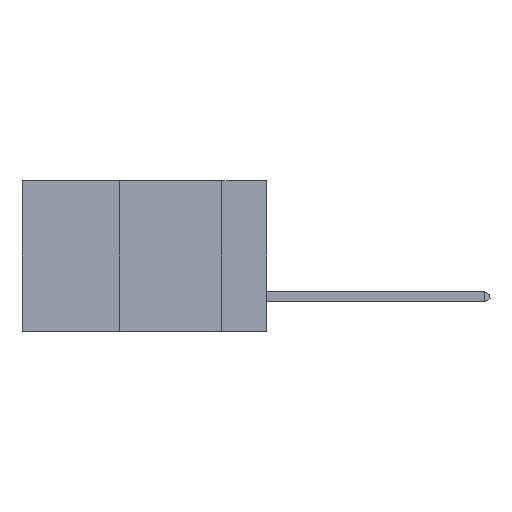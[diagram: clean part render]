
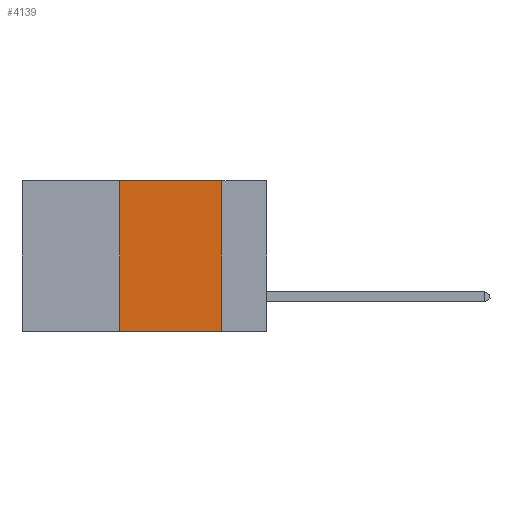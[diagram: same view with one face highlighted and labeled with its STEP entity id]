
A CAD part, left-side view. The second image highlights one B-rep face of the part: STEP entity #4139.
In plain terms, the highlighted planar face has unit normal (-1, 0, 0).
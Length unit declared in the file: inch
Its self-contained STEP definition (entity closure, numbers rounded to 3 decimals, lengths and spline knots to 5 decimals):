
#170 = LINE ( 'NONE', #10592, #1726 ) ;
#188 = ORIENTED_EDGE ( 'NONE', *, *, #2521, .F. ) ;
#624 = DIRECTION ( 'NONE',  ( 0., 0., 1. ) ) ;
#877 = VERTEX_POINT ( 'NONE', #3341 ) ;
#1726 = VECTOR ( 'NONE', #624, 39.37008 ) ;
#2051 = EDGE_CURVE ( 'NONE', #2787, #7025, #6149, .T. ) ;
#2108 = PLANE ( 'NONE',  #3985 ) ;
#2503 = ORIENTED_EDGE ( 'NONE', *, *, #2051, .T. ) ;
#2521 = EDGE_CURVE ( 'NONE', #2787, #10361, #170, .T. ) ;
#2787 = VERTEX_POINT ( 'NONE', #4578 ) ;
#2867 = CARTESIAN_POINT ( 'NONE',  ( 0., 0.6, 0. ) ) ;
#3189 = VECTOR ( 'NONE', #7987, 39.37008 ) ;
#3257 = EDGE_CURVE ( 'NONE', #877, #7025, #10540, .T. ) ;
#3341 = CARTESIAN_POINT ( 'NONE',  ( 0., 0.11, 0. ) ) ;
#3731 = EDGE_LOOP ( 'NONE', ( #8796, #10254, #188, #2503 ) ) ;
#3985 = AXIS2_PLACEMENT_3D ( 'NONE', #2867, #7117, #4519 ) ;
#4139 = ADVANCED_FACE ( 'NONE', ( #6765 ), #2108, .F. ) ;
#4481 = VECTOR ( 'NONE', #10530, 39.37008 ) ;
#4519 = DIRECTION ( 'NONE',  ( 0., 0., -1. ) ) ;
#4578 = CARTESIAN_POINT ( 'NONE',  ( 0., 0.36, -0.37 ) ) ;
#4803 = CARTESIAN_POINT ( 'NONE',  ( 0., 0.11, 0. ) ) ;
#4888 = VECTOR ( 'NONE', #7422, 39.37008 ) ;
#5775 = CARTESIAN_POINT ( 'NONE',  ( 0., 0.6, 0. ) ) ;
#6149 = LINE ( 'NONE', #9600, #3189 ) ;
#6765 = FACE_OUTER_BOUND ( 'NONE', #3731, .T. ) ;
#6956 = CARTESIAN_POINT ( 'NONE',  ( 0., 0.11, -0.37 ) ) ;
#7025 = VERTEX_POINT ( 'NONE', #6956 ) ;
#7117 = DIRECTION ( 'NONE',  ( 1., 0., 0. ) ) ;
#7422 = DIRECTION ( 'NONE',  ( 0., -1., 0. ) ) ;
#7870 = LINE ( 'NONE', #5775, #4888 ) ;
#7987 = DIRECTION ( 'NONE',  ( 0., -1., 0. ) ) ;
#8382 = EDGE_CURVE ( 'NONE', #10361, #877, #7870, .T. ) ;
#8796 = ORIENTED_EDGE ( 'NONE', *, *, #3257, .F. ) ;
#8949 = CARTESIAN_POINT ( 'NONE',  ( 0., 0.36, 0. ) ) ;
#9600 = CARTESIAN_POINT ( 'NONE',  ( 0., 0.6, -0.37 ) ) ;
#10254 = ORIENTED_EDGE ( 'NONE', *, *, #8382, .F. ) ;
#10361 = VERTEX_POINT ( 'NONE', #8949 ) ;
#10530 = DIRECTION ( 'NONE',  ( 0., 0., -1. ) ) ;
#10540 = LINE ( 'NONE', #4803, #4481 ) ;
#10592 = CARTESIAN_POINT ( 'NONE',  ( 0., 0.36, 0. ) ) ;
